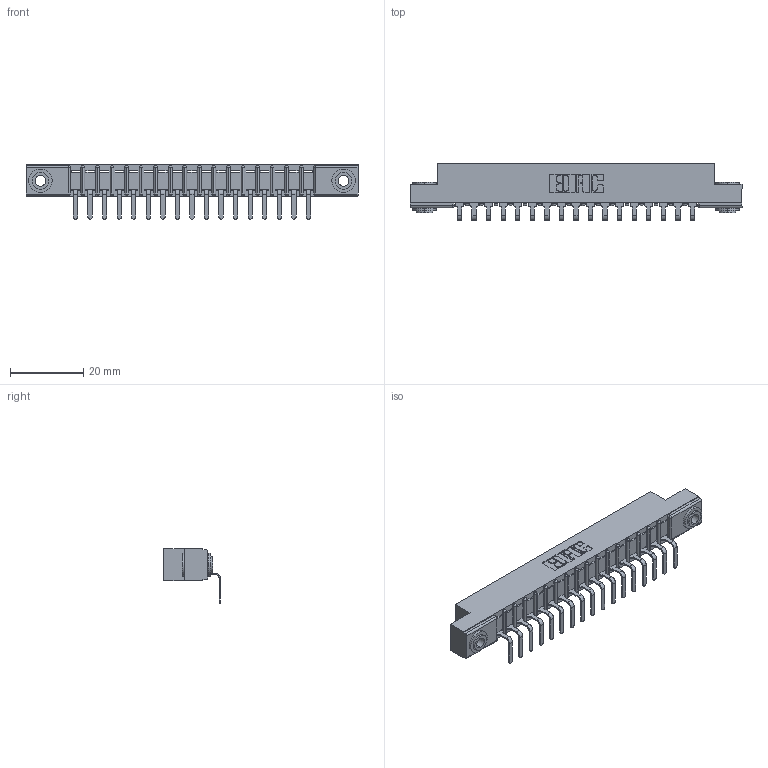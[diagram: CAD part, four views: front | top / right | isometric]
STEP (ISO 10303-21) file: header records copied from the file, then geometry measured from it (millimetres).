
FILE_DESCRIPTION (( 'STEP AP203' ), '1' );
FILE_NAME ('307-017-559-103.STEP', '2019-09-04T16:01:02', ( '' ), ( '' ), 'SwSTEP 2.0', 'SolidWorks 2016', '' );
FILE_SCHEMA (( 'CONFIG_CONTROL_DESIGN' ));
Length unit declared in the file: inch
Products named in the file (4): 345-250-002_345-250-002-102; 307 Part_.156 Dia Mounting Holes; 307-017-559-103; 307-290-001_558 559 - 1 (Single)
Assembly tree (20 placements, depth 2):
  307-017-559-103
    307 Part_.156 Dia Mounting Holes
    307-290-001_558 559 - 1 (Single)  x17
    345-250-002_345-250-002-102  x2
Bounding box: 90.37 x 15.46 x 14.81 mm (x, y, z)
Volume: 5740.3 mm3; surface area: 9080.8 mm2
Topology: 20 solids, 20 shells, 1208 faces, 3393 edges, 2186 vertices
Faces by surface type: plane 757, cylinder 407, sphere 36, cone 8
Entity records: 18825 total; most frequent: CARTESIAN_POINT 3141, ORIENTED_EDGE 3118, DIRECTION 3085, EDGE_CURVE 1559, VECTOR 1177, LINE 1177, VERTEX_POINT 1010, AXIS2_PLACEMENT_3D 954
